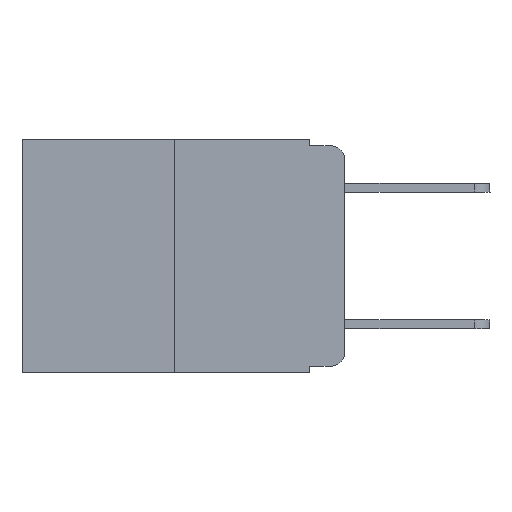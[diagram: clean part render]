
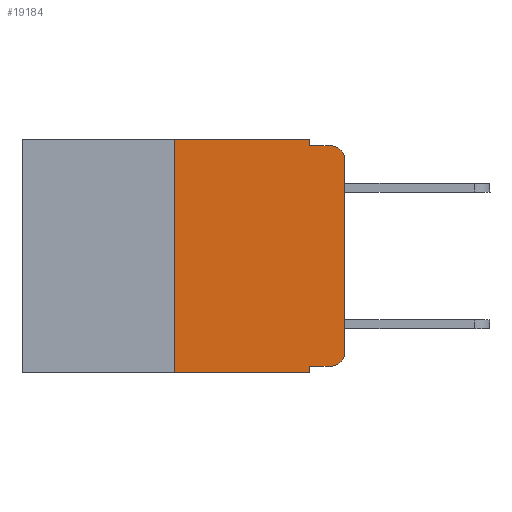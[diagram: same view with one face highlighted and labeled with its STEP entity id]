
A CAD part, left-side view. The second image highlights one B-rep face of the part: STEP entity #19184.
In plain terms, the highlighted planar face has unit normal (-1, 0, 0).
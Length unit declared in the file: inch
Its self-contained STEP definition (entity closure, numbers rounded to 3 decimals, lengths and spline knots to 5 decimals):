
#18 = FACE_OUTER_BOUND ( 'NONE', #14011, .T. ) ;
#43 = CARTESIAN_POINT ( 'NONE',  ( 0., 0.25, 0. ) ) ;
#441 = VECTOR ( 'NONE', #23192, 39.37008 ) ;
#513 = ORIENTED_EDGE ( 'NONE', *, *, #7770, .F. ) ;
#904 = AXIS2_PLACEMENT_3D ( 'NONE', #7531, #5689, #13431 ) ;
#931 = VECTOR ( 'NONE', #17208, 39.37008 ) ;
#1023 = EDGE_CURVE ( 'NONE', #18883, #16447, #17589, .T. ) ;
#1413 = CIRCLE ( 'NONE', #9658, 0.02 ) ;
#1988 = DIRECTION ( 'NONE',  ( 0., 0., 1. ) ) ;
#2090 = DIRECTION ( 'NONE',  ( 0., 0., -1. ) ) ;
#2156 = VECTOR ( 'NONE', #22097, 39.37008 ) ;
#2903 = ORIENTED_EDGE ( 'NONE', *, *, #22765, .T. ) ;
#3469 = DIRECTION ( 'NONE',  ( -1., 0., 0. ) ) ;
#3719 = DIRECTION ( 'NONE',  ( 0., 0., -1. ) ) ;
#3812 = DIRECTION ( 'NONE',  ( 0., 0., 1. ) ) ;
#4053 = EDGE_CURVE ( 'NONE', #7246, #6002, #7852, .T. ) ;
#4077 = VERTEX_POINT ( 'NONE', #11562 ) ;
#5000 = VERTEX_POINT ( 'NONE', #22680 ) ;
#5689 = DIRECTION ( 'NONE',  ( 1., 0., 0. ) ) ;
#5892 = DIRECTION ( 'NONE',  ( 0., -1., 0. ) ) ;
#6002 = VERTEX_POINT ( 'NONE', #8155 ) ;
#6352 = VECTOR ( 'NONE', #3812, 39.37008 ) ;
#6400 = CARTESIAN_POINT ( 'NONE',  ( 0., 0.02, -0.313 ) ) ;
#6686 = CARTESIAN_POINT ( 'NONE',  ( 0., 0.02, -0.333 ) ) ;
#7246 = VERTEX_POINT ( 'NONE', #19541 ) ;
#7361 = ORIENTED_EDGE ( 'NONE', *, *, #11290, .F. ) ;
#7531 = CARTESIAN_POINT ( 'NONE',  ( 0., 0.473, 0. ) ) ;
#7770 = EDGE_CURVE ( 'NONE', #15010, #9439, #10048, .T. ) ;
#7852 = LINE ( 'NONE', #11684, #21362 ) ;
#8155 = CARTESIAN_POINT ( 'NONE',  ( 0., 0.02, -0.01 ) ) ;
#8942 = CARTESIAN_POINT ( 'NONE',  ( 0., 0.051, -0.333 ) ) ;
#9439 = VERTEX_POINT ( 'NONE', #17262 ) ;
#9475 = LINE ( 'NONE', #18932, #931 ) ;
#9658 = AXIS2_PLACEMENT_3D ( 'NONE', #15160, #3469, #3719 ) ;
#9982 = ORIENTED_EDGE ( 'NONE', *, *, #1023, .T. ) ;
#10048 = LINE ( 'NONE', #17535, #441 ) ;
#10383 = EDGE_CURVE ( 'NONE', #15570, #4077, #13534, .T. ) ;
#10437 = EDGE_CURVE ( 'NONE', #17388, #9439, #9475, .T. ) ;
#10760 = VECTOR ( 'NONE', #5892, 39.37008 ) ;
#11290 = EDGE_CURVE ( 'NONE', #17388, #15570, #20945, .T. ) ;
#11444 = LINE ( 'NONE', #18931, #14670 ) ;
#11562 = CARTESIAN_POINT ( 'NONE',  ( 0., 0.051, 0. ) ) ;
#11684 = CARTESIAN_POINT ( 'NONE',  ( 0., 0.051, -0.01 ) ) ;
#12106 = AXIS2_PLACEMENT_3D ( 'NONE', #6400, #17470, #23127 ) ;
#13174 = LINE ( 'NONE', #20667, #6352 ) ;
#13431 = DIRECTION ( 'NONE',  ( 0., 0., -1. ) ) ;
#13534 = LINE ( 'NONE', #15250, #10760 ) ;
#14011 = EDGE_LOOP ( 'NONE', ( #19261, #23394, #15461, #22482, #20593, #7361, #14337, #513, #2903, #9982 ) ) ;
#14337 = ORIENTED_EDGE ( 'NONE', *, *, #10437, .T. ) ;
#14670 = VECTOR ( 'NONE', #2090, 39.37008 ) ;
#14911 = VECTOR ( 'NONE', #1988, 39.37008 ) ;
#15010 = VERTEX_POINT ( 'NONE', #23730 ) ;
#15160 = CARTESIAN_POINT ( 'NONE',  ( 0., 0.02, -0.03 ) ) ;
#15169 = CARTESIAN_POINT ( 'NONE',  ( 0., 0.25, 0. ) ) ;
#15250 = CARTESIAN_POINT ( 'NONE',  ( 0., 0.473, 0. ) ) ;
#15352 = DIRECTION ( 'NONE',  ( 0., -1., 0. ) ) ;
#15461 = ORIENTED_EDGE ( 'NONE', *, *, #4053, .F. ) ;
#15570 = VERTEX_POINT ( 'NONE', #43 ) ;
#16058 = EDGE_CURVE ( 'NONE', #5000, #6002, #1413, .T. ) ;
#16447 = VERTEX_POINT ( 'NONE', #17178 ) ;
#17003 = PLANE ( 'NONE',  #904 ) ;
#17178 = CARTESIAN_POINT ( 'NONE',  ( 0., 0., -0.313 ) ) ;
#17208 = DIRECTION ( 'NONE',  ( 0., -1., 0. ) ) ;
#17262 = CARTESIAN_POINT ( 'NONE',  ( 0., 0.051, -0.343 ) ) ;
#17388 = VERTEX_POINT ( 'NONE', #20693 ) ;
#17470 = DIRECTION ( 'NONE',  ( -1., 0., 0. ) ) ;
#17535 = CARTESIAN_POINT ( 'NONE',  ( 0., 0.051, 0. ) ) ;
#17589 = CIRCLE ( 'NONE', #12106, 0.02 ) ;
#17894 = EDGE_CURVE ( 'NONE', #16447, #5000, #13174, .T. ) ;
#18883 = VERTEX_POINT ( 'NONE', #6686 ) ;
#18931 = CARTESIAN_POINT ( 'NONE',  ( 0., 0.051, 0. ) ) ;
#18932 = CARTESIAN_POINT ( 'NONE',  ( 0., 0.473, -0.343 ) ) ;
#19184 = ADVANCED_FACE ( 'NONE', ( #18 ), #17003, .F. ) ;
#19261 = ORIENTED_EDGE ( 'NONE', *, *, #17894, .T. ) ;
#19541 = CARTESIAN_POINT ( 'NONE',  ( 0., 0.051, -0.01 ) ) ;
#19589 = EDGE_CURVE ( 'NONE', #4077, #7246, #11444, .T. ) ;
#19781 = LINE ( 'NONE', #8942, #2156 ) ;
#20593 = ORIENTED_EDGE ( 'NONE', *, *, #10383, .F. ) ;
#20667 = CARTESIAN_POINT ( 'NONE',  ( 0., 0., 0. ) ) ;
#20693 = CARTESIAN_POINT ( 'NONE',  ( 0., 0.25, -0.343 ) ) ;
#20945 = LINE ( 'NONE', #15169, #14911 ) ;
#21362 = VECTOR ( 'NONE', #15352, 39.37008 ) ;
#22097 = DIRECTION ( 'NONE',  ( 0., -1., 0. ) ) ;
#22482 = ORIENTED_EDGE ( 'NONE', *, *, #19589, .F. ) ;
#22680 = CARTESIAN_POINT ( 'NONE',  ( 0., 0., -0.03 ) ) ;
#22765 = EDGE_CURVE ( 'NONE', #15010, #18883, #19781, .T. ) ;
#23127 = DIRECTION ( 'NONE',  ( 0., 0., -1. ) ) ;
#23192 = DIRECTION ( 'NONE',  ( 0., 0., -1. ) ) ;
#23394 = ORIENTED_EDGE ( 'NONE', *, *, #16058, .T. ) ;
#23730 = CARTESIAN_POINT ( 'NONE',  ( 0., 0.051, -0.333 ) ) ;
